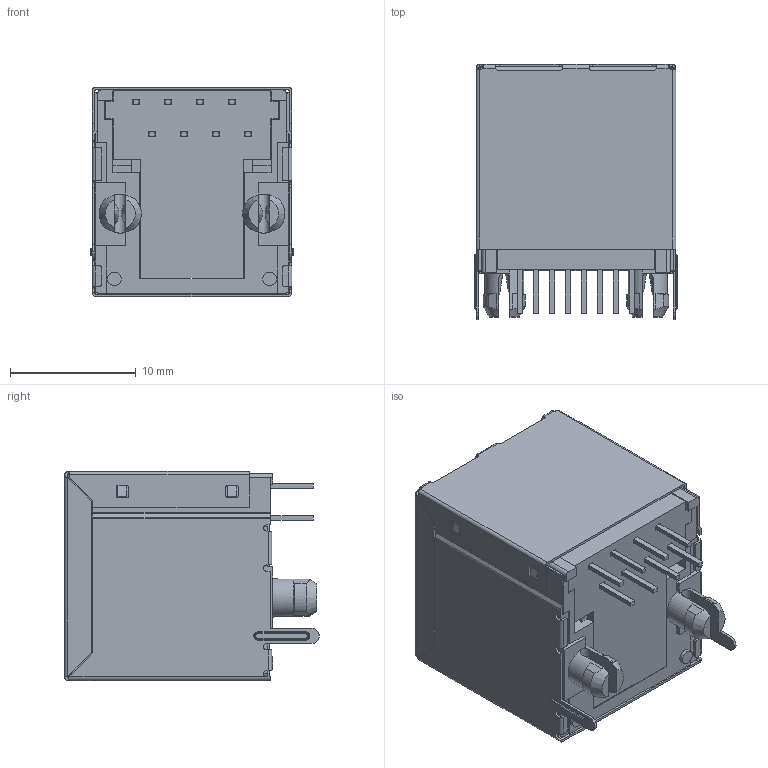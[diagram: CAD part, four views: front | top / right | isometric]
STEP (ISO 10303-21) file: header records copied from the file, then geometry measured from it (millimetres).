
FILE_DESCRIPTION (( 'STEP AP203' ), '1' );
FILE_NAME ('RJ2L018891P00131.STEP', '2019-12-16T14:21:40', ( '' ), ( '' ), 'SwSTEP 2.0', 'SolidWorks 2016', '' );
FILE_SCHEMA (( 'CONFIG_CONTROL_DESIGN' ));
Length unit declared in the file: millimetre
Products named in the file (5): RJ2L018891P00131; 2L Shield; 2L Contacts; 2L Insulator; 2L Contact Lock
Assembly tree (4 placements, depth 2):
  RJ2L018891P00131
    2L Insulator
    2L Contacts
    2L Contact Lock
    2L Shield
Bounding box: 16.2 x 20.3 x 16.65 mm (x, y, z)
Volume: 2717.1 mm3; surface area: 6472.8 mm2
Topology: 11 solids, 11 shells, 1125 faces, 3168 edges, 2043 vertices
Faces by surface type: plane 778, cylinder 284, bspline 55, cone 8
Entity records: 37977 total; most frequent: CARTESIAN_POINT 9112, ORIENTED_EDGE 6320, DIRECTION 5323, EDGE_CURVE 3160, VECTOR 2443, LINE 2443, VERTEX_POINT 2043, AXIS2_PLACEMENT_3D 1440
